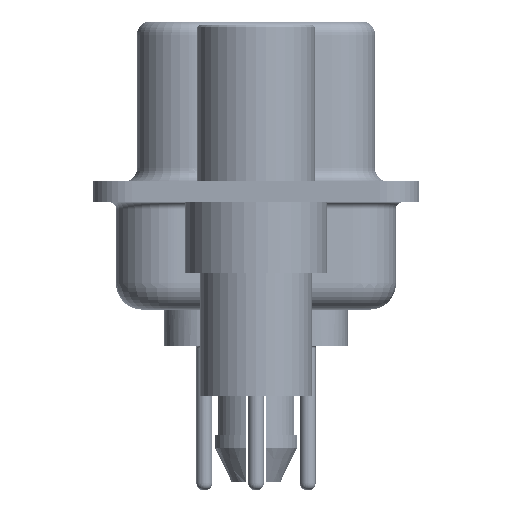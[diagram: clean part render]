
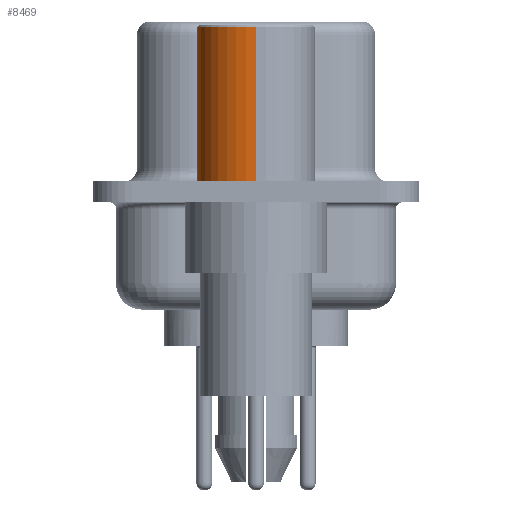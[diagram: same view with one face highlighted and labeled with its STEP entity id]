
A CAD part, left-side view. The second image highlights one B-rep face of the part: STEP entity #8469.
In plain terms, the highlighted cylindrical face has radius 2.25 mm (diameter 4.5 mm), a partial arc.
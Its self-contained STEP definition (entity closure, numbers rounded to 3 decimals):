
#345 = VECTOR ( 'NONE', #20647, 1000. ) ;
#1852 = EDGE_CURVE ( 'NONE', #24752, #25757, #7079, .T. ) ;
#3247 = FACE_OUTER_BOUND ( 'NONE', #3986, .T. ) ;
#3986 = EDGE_LOOP ( 'NONE', ( #31982, #29151, #9472, #33265 ) ) ;
#4020 = DIRECTION ( 'NONE',  ( 0., 0., 1. ) ) ;
#6779 = CARTESIAN_POINT ( 'NONE',  ( 2.25, 0., 0.4 ) ) ;
#7079 = LINE ( 'NONE', #15257, #26790 ) ;
#7494 = CARTESIAN_POINT ( 'NONE',  ( 2.25, 0., 6.3 ) ) ;
#8149 = CARTESIAN_POINT ( 'NONE',  ( -2.25, 0., 6.3 ) ) ;
#8469 = ADVANCED_FACE ( 'NONE', ( #3247 ), #16272, .T. ) ;
#9254 = CARTESIAN_POINT ( 'NONE',  ( -2.25, 0., 0.4 ) ) ;
#9472 = ORIENTED_EDGE ( 'NONE', *, *, #29538, .F. ) ;
#10127 = AXIS2_PLACEMENT_3D ( 'NONE', #19550, #4020, #22122 ) ;
#11928 = DIRECTION ( 'NONE',  ( 1., 0., 0. ) ) ;
#12682 = DIRECTION ( 'NONE',  ( 0., 0., 1. ) ) ;
#13137 = CIRCLE ( 'NONE', #10127, 2.25 ) ;
#13832 = VERTEX_POINT ( 'NONE', #7494 ) ;
#15257 = CARTESIAN_POINT ( 'NONE',  ( -2.25, 0., 0.581 ) ) ;
#16173 = AXIS2_PLACEMENT_3D ( 'NONE', #28039, #12682, #30579 ) ;
#16272 = CYLINDRICAL_SURFACE ( 'NONE', #23340, 2.25 ) ;
#19140 = VERTEX_POINT ( 'NONE', #6779 ) ;
#19295 = EDGE_CURVE ( 'NONE', #19140, #24752, #19465, .T. ) ;
#19465 = CIRCLE ( 'NONE', #16173, 2.25 ) ;
#19550 = CARTESIAN_POINT ( 'NONE',  ( 0., 0., 6.3 ) ) ;
#19923 = EDGE_CURVE ( 'NONE', #19140, #13832, #27895, .T. ) ;
#20647 = DIRECTION ( 'NONE',  ( 0., 0., 1. ) ) ;
#20727 = DIRECTION ( 'NONE',  ( 0., 0., 1. ) ) ;
#22122 = DIRECTION ( 'NONE',  ( 1., 0., 0. ) ) ;
#23340 = AXIS2_PLACEMENT_3D ( 'NONE', #29837, #24711, #11928 ) ;
#24711 = DIRECTION ( 'NONE',  ( 0., 0., 1. ) ) ;
#24752 = VERTEX_POINT ( 'NONE', #9254 ) ;
#25757 = VERTEX_POINT ( 'NONE', #8149 ) ;
#26790 = VECTOR ( 'NONE', #20727, 1000. ) ;
#27895 = LINE ( 'NONE', #30779, #345 ) ;
#28039 = CARTESIAN_POINT ( 'NONE',  ( 0., 0., 0.4 ) ) ;
#29151 = ORIENTED_EDGE ( 'NONE', *, *, #1852, .T. ) ;
#29538 = EDGE_CURVE ( 'NONE', #13832, #25757, #13137, .T. ) ;
#29837 = CARTESIAN_POINT ( 'NONE',  ( 0., 0., 0.581 ) ) ;
#30579 = DIRECTION ( 'NONE',  ( 1., 0., 0. ) ) ;
#30779 = CARTESIAN_POINT ( 'NONE',  ( 2.25, 0., 0.581 ) ) ;
#31982 = ORIENTED_EDGE ( 'NONE', *, *, #19295, .T. ) ;
#33265 = ORIENTED_EDGE ( 'NONE', *, *, #19923, .F. ) ;
